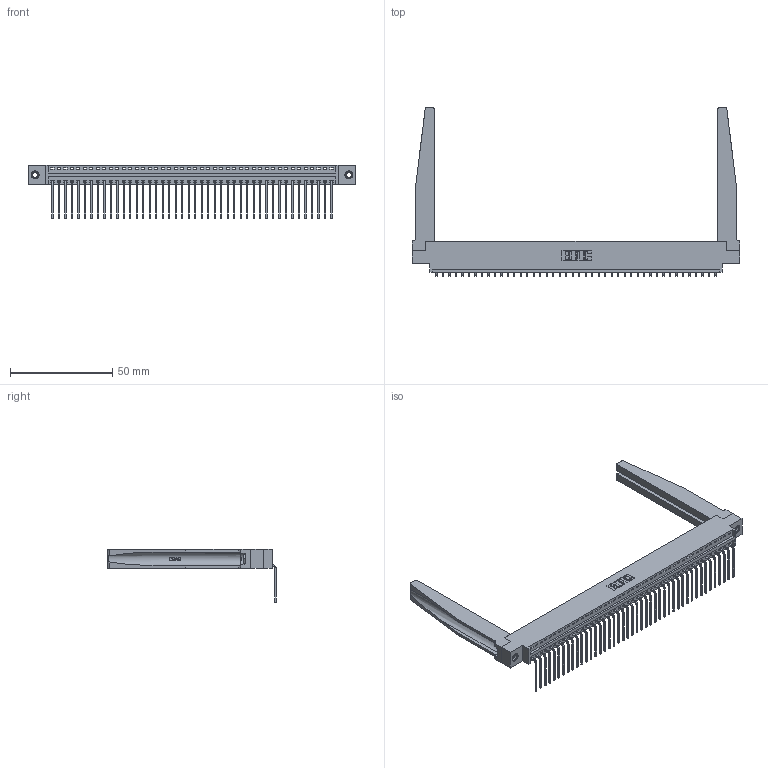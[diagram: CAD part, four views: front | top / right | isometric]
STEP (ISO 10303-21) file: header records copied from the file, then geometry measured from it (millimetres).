
FILE_DESCRIPTION (( 'STEP AP203' ), '1' );
FILE_NAME ('346-044-559-678.STEP', '2022-05-09T17:50:21', ( '' ), ( '' ), 'SwSTEP 2.0', 'SolidWorks 2020', '' );
FILE_SCHEMA (( 'CONFIG_CONTROL_DESIGN' ));
Length unit declared in the file: inch
Products named in the file (5): 345-292-001_558 559 Tail - 1; 345-250-001_345-250-001-102; 346 Part_0.170 Offset - 0.156 Dia-TH; 346-044-559-678; 346-220-078_345-220-078
Assembly tree (49 placements, depth 2):
  346-044-559-678
    346 Part_0.170 Offset - 0.156 Dia-TH
    345-292-001_558 559 Tail - 1  x44
    346-220-078_345-220-078  x2
    345-250-001_345-250-001-102  x2
Bounding box: 160.27 x 82.36 x 26.16 mm (x, y, z)
Volume: 22238.3 mm3; surface area: 26788.7 mm2
Topology: 49 solids, 49 shells, 3014 faces, 8993 edges, 5926 vertices
Faces by surface type: plane 2084, cylinder 878, bspline 36, cone 12, torus 4
Entity records: 32418 total; most frequent: CARTESIAN_POINT 6473, ORIENTED_EDGE 5338, DIRECTION 4691, EDGE_CURVE 2669, LINE 2267, VECTOR 2267, VERTEX_POINT 1772, AXIS2_PLACEMENT_3D 1212
